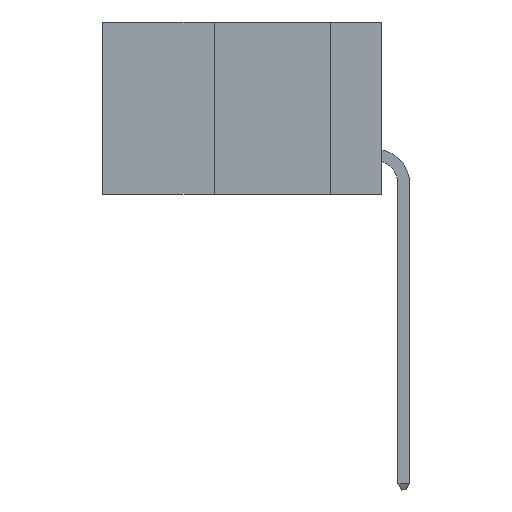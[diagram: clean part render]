
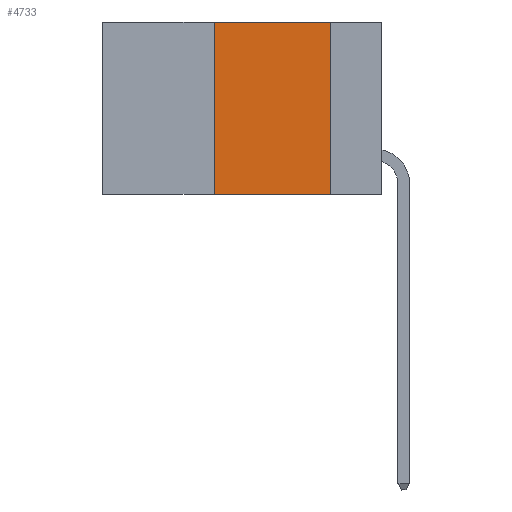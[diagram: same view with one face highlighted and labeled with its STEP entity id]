
A CAD part, left-side view. The second image highlights one B-rep face of the part: STEP entity #4733.
In plain terms, the highlighted planar face has unit normal (-1, 0, 0).
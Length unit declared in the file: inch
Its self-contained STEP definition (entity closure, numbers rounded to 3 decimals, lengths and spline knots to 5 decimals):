
#450 = CARTESIAN_POINT ( 'NONE',  ( 0., 0.36, 0. ) ) ;
#490 = CARTESIAN_POINT ( 'NONE',  ( 0., 0.36, 0. ) ) ;
#577 = ORIENTED_EDGE ( 'NONE', *, *, #845, .F. ) ;
#845 = EDGE_CURVE ( 'NONE', #4179, #18297, #1950, .T. ) ;
#1074 = CARTESIAN_POINT ( 'NONE',  ( 0., 0.11, 0. ) ) ;
#1934 = PLANE ( 'NONE',  #9158 ) ;
#1950 = LINE ( 'NONE', #490, #15704 ) ;
#2415 = EDGE_CURVE ( 'NONE', #4179, #19655, #4367, .T. ) ;
#3043 = EDGE_CURVE ( 'NONE', #7048, #19655, #13355, .T. ) ;
#3546 = ORIENTED_EDGE ( 'NONE', *, *, #3043, .F. ) ;
#3871 = EDGE_CURVE ( 'NONE', #18297, #7048, #16506, .T. ) ;
#4054 = CARTESIAN_POINT ( 'NONE',  ( 0., 0.11, 0. ) ) ;
#4179 = VERTEX_POINT ( 'NONE', #12620 ) ;
#4327 = VECTOR ( 'NONE', #6050, 39.37008 ) ;
#4367 = LINE ( 'NONE', #4699, #5388 ) ;
#4699 = CARTESIAN_POINT ( 'NONE',  ( 0., 0.6, -0.37 ) ) ;
#4733 = ADVANCED_FACE ( 'NONE', ( #7987 ), #1934, .F. ) ;
#4824 = DIRECTION ( 'NONE',  ( 0., -1., 0. ) ) ;
#5305 = CARTESIAN_POINT ( 'NONE',  ( 0., 0.6, 0. ) ) ;
#5388 = VECTOR ( 'NONE', #4824, 39.37008 ) ;
#6050 = DIRECTION ( 'NONE',  ( 0., 0., -1. ) ) ;
#6919 = DIRECTION ( 'NONE',  ( 0., 0., 1. ) ) ;
#7048 = VERTEX_POINT ( 'NONE', #4054 ) ;
#7987 = FACE_OUTER_BOUND ( 'NONE', #13939, .T. ) ;
#9158 = AXIS2_PLACEMENT_3D ( 'NONE', #19190, #17662, #15220 ) ;
#10127 = DIRECTION ( 'NONE',  ( 0., -1., 0. ) ) ;
#11241 = ORIENTED_EDGE ( 'NONE', *, *, #3871, .F. ) ;
#11487 = VECTOR ( 'NONE', #10127, 39.37008 ) ;
#12620 = CARTESIAN_POINT ( 'NONE',  ( 0., 0.36, -0.37 ) ) ;
#13214 = CARTESIAN_POINT ( 'NONE',  ( 0., 0.11, -0.37 ) ) ;
#13355 = LINE ( 'NONE', #1074, #4327 ) ;
#13939 = EDGE_LOOP ( 'NONE', ( #3546, #11241, #577, #15816 ) ) ;
#15220 = DIRECTION ( 'NONE',  ( 0., 0., -1. ) ) ;
#15704 = VECTOR ( 'NONE', #6919, 39.37008 ) ;
#15816 = ORIENTED_EDGE ( 'NONE', *, *, #2415, .T. ) ;
#16506 = LINE ( 'NONE', #5305, #11487 ) ;
#17662 = DIRECTION ( 'NONE',  ( 1., 0., 0. ) ) ;
#18297 = VERTEX_POINT ( 'NONE', #450 ) ;
#19190 = CARTESIAN_POINT ( 'NONE',  ( 0., 0.6, 0. ) ) ;
#19655 = VERTEX_POINT ( 'NONE', #13214 ) ;
